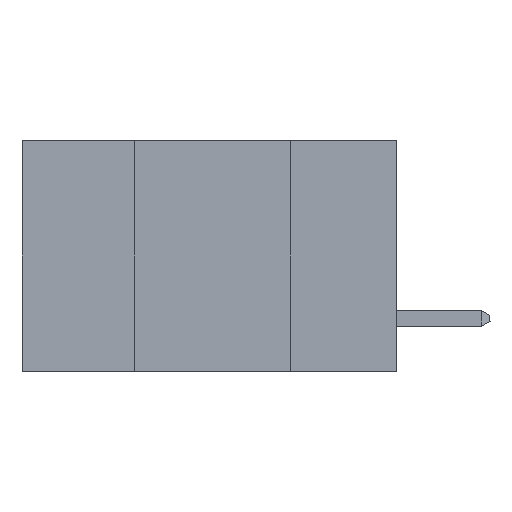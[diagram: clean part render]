
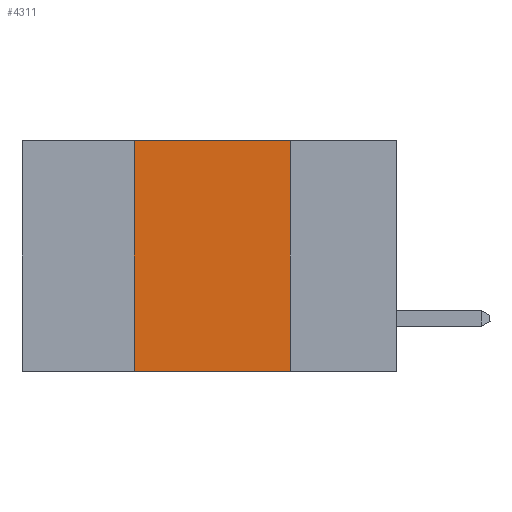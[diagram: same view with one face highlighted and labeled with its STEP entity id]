
A CAD part, left-side view. The second image highlights one B-rep face of the part: STEP entity #4311.
In plain terms, the highlighted planar face has unit normal (-1, 0, 0).
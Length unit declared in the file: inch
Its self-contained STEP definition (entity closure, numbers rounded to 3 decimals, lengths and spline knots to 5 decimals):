
#12 = CARTESIAN_POINT ( 'NONE',  ( 0., 0.17, 0. ) ) ;
#797 = ORIENTED_EDGE ( 'NONE', *, *, #7975, .F. ) ;
#864 = CARTESIAN_POINT ( 'NONE',  ( 0., 0.17, 0. ) ) ;
#2503 = PLANE ( 'NONE',  #11167 ) ;
#2668 = LINE ( 'NONE', #864, #10265 ) ;
#3897 = VECTOR ( 'NONE', #9575, 39.37008 ) ;
#3970 = DIRECTION ( 'NONE',  ( 1., 0., 0. ) ) ;
#4311 = ADVANCED_FACE ( 'NONE', ( #6066 ), #2503, .F. ) ;
#5180 = CARTESIAN_POINT ( 'NONE',  ( 0., 0.42, -0.37 ) ) ;
#5404 = DIRECTION ( 'NONE',  ( 0., 0., -1. ) ) ;
#5549 = EDGE_CURVE ( 'NONE', #12911, #16709, #16104, .T. ) ;
#6066 = FACE_OUTER_BOUND ( 'NONE', #15722, .T. ) ;
#7450 = EDGE_CURVE ( 'NONE', #10744, #16709, #2668, .T. ) ;
#7632 = CARTESIAN_POINT ( 'NONE',  ( 0., 0.6, -0.37 ) ) ;
#7975 = EDGE_CURVE ( 'NONE', #12911, #14201, #15591, .T. ) ;
#8103 = VECTOR ( 'NONE', #9072, 39.37008 ) ;
#9072 = DIRECTION ( 'NONE',  ( 0., -1., 0. ) ) ;
#9174 = DIRECTION ( 'NONE',  ( 0., 0., -1. ) ) ;
#9224 = CARTESIAN_POINT ( 'NONE',  ( 0., 0.42, 0. ) ) ;
#9575 = DIRECTION ( 'NONE',  ( 0., -1., 0. ) ) ;
#10265 = VECTOR ( 'NONE', #9174, 39.37008 ) ;
#10744 = VERTEX_POINT ( 'NONE', #12 ) ;
#11167 = AXIS2_PLACEMENT_3D ( 'NONE', #15339, #3970, #5404 ) ;
#11514 = ORIENTED_EDGE ( 'NONE', *, *, #18042, .F. ) ;
#12697 = CARTESIAN_POINT ( 'NONE',  ( 0., 0.6, 0. ) ) ;
#12706 = VECTOR ( 'NONE', #15366, 39.37008 ) ;
#12751 = ORIENTED_EDGE ( 'NONE', *, *, #7450, .F. ) ;
#12911 = VERTEX_POINT ( 'NONE', #5180 ) ;
#14015 = CARTESIAN_POINT ( 'NONE',  ( 0., 0.42, 0. ) ) ;
#14201 = VERTEX_POINT ( 'NONE', #9224 ) ;
#15339 = CARTESIAN_POINT ( 'NONE',  ( 0., 0.6, 0. ) ) ;
#15366 = DIRECTION ( 'NONE',  ( 0., 0., 1. ) ) ;
#15591 = LINE ( 'NONE', #14015, #12706 ) ;
#15722 = EDGE_LOOP ( 'NONE', ( #12751, #11514, #797, #16992 ) ) ;
#15793 = CARTESIAN_POINT ( 'NONE',  ( 0., 0.17, -0.37 ) ) ;
#16104 = LINE ( 'NONE', #7632, #8103 ) ;
#16709 = VERTEX_POINT ( 'NONE', #15793 ) ;
#16992 = ORIENTED_EDGE ( 'NONE', *, *, #5549, .T. ) ;
#17667 = LINE ( 'NONE', #12697, #3897 ) ;
#18042 = EDGE_CURVE ( 'NONE', #14201, #10744, #17667, .T. ) ;
